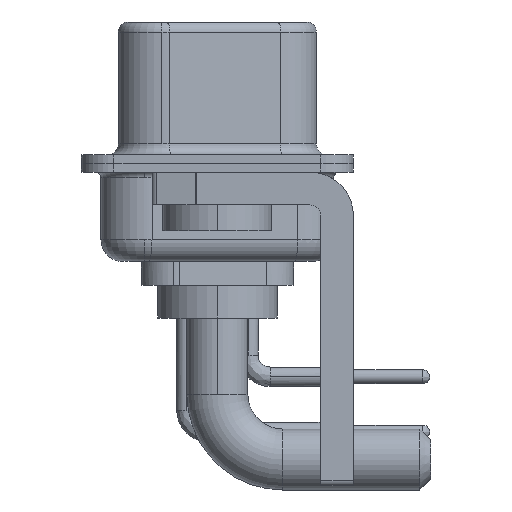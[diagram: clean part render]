
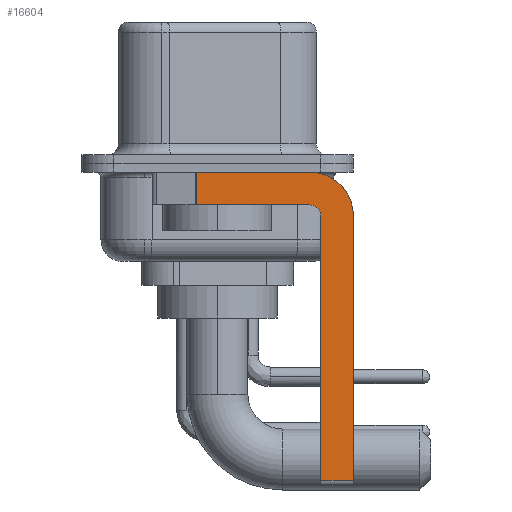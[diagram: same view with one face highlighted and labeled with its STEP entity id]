
A CAD part, left-side view. The second image highlights one B-rep face of the part: STEP entity #16604.
In plain terms, the highlighted planar face has unit normal (-1, 0, 0).
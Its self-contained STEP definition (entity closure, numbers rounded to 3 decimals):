
#209 = LINE ( 'NONE', #8824, #12988 ) ;
#269 = CARTESIAN_POINT ( 'NONE',  ( -2.9, 3., -0.4 ) ) ;
#387 = DIRECTION ( 'NONE',  ( 0., -1., 0. ) ) ;
#455 = DIRECTION ( 'NONE',  ( -1., 0., 0. ) ) ;
#853 = VECTOR ( 'NONE', #387, 1000. ) ;
#1752 = DIRECTION ( 'NONE',  ( 1., 0., 0. ) ) ;
#2207 = DIRECTION ( 'NONE',  ( 0., 0., -1. ) ) ;
#2920 = ORIENTED_EDGE ( 'NONE', *, *, #16325, .F. ) ;
#2950 = VERTEX_POINT ( 'NONE', #22799 ) ;
#3024 = FACE_OUTER_BOUND ( 'NONE', #8838, .T. ) ;
#3035 = CARTESIAN_POINT ( 'NONE',  ( -2.9, 0.978, -0.4 ) ) ;
#3582 = VERTEX_POINT ( 'NONE', #8939 ) ;
#3857 = LINE ( 'NONE', #11533, #7801 ) ;
#3875 = LINE ( 'NONE', #12969, #11647 ) ;
#4108 = ORIENTED_EDGE ( 'NONE', *, *, #15287, .F. ) ;
#4425 = DIRECTION ( 'NONE',  ( 0., 0., 1. ) ) ;
#4840 = CARTESIAN_POINT ( 'NONE',  ( -2.9, 0.978, -1.9 ) ) ;
#4851 = AXIS2_PLACEMENT_3D ( 'NONE', #7416, #1752, #12620 ) ;
#5458 = EDGE_CURVE ( 'NONE', #9371, #8896, #209, .T. ) ;
#5978 = VERTEX_POINT ( 'NONE', #4840 ) ;
#6232 = ORIENTED_EDGE ( 'NONE', *, *, #9484, .T. ) ;
#6347 = ORIENTED_EDGE ( 'NONE', *, *, #21691, .F. ) ;
#6427 = CARTESIAN_POINT ( 'NONE',  ( -2.9, -4.75, -14.8 ) ) ;
#6877 = LINE ( 'NONE', #15976, #7478 ) ;
#7175 = DIRECTION ( 'NONE',  ( 0., 0., 1. ) ) ;
#7180 = DIRECTION ( 'NONE',  ( 0., 1., 0. ) ) ;
#7416 = CARTESIAN_POINT ( 'NONE',  ( -2.9, -4.25, -2.4 ) ) ;
#7478 = VECTOR ( 'NONE', #14556, 1000. ) ;
#7801 = VECTOR ( 'NONE', #2207, 1000. ) ;
#8552 = ORIENTED_EDGE ( 'NONE', *, *, #16240, .F. ) ;
#8640 = VECTOR ( 'NONE', #4425, 1000. ) ;
#8824 = CARTESIAN_POINT ( 'NONE',  ( -2.9, -6.25, -2.4 ) ) ;
#8838 = EDGE_LOOP ( 'NONE', ( #4108, #6232, #8552, #6347, #14166, #11772, #13101, #2920 ) ) ;
#8896 = VERTEX_POINT ( 'NONE', #14082 ) ;
#8939 = CARTESIAN_POINT ( 'NONE',  ( -2.9, -4.75, -14.55 ) ) ;
#9371 = VERTEX_POINT ( 'NONE', #10715 ) ;
#9484 = EDGE_CURVE ( 'NONE', #19626, #5978, #3857, .T. ) ;
#10115 = DIRECTION ( 'NONE',  ( 0., 0., -1. ) ) ;
#10374 = EDGE_CURVE ( 'NONE', #3582, #8896, #6877, .T. ) ;
#10464 = CARTESIAN_POINT ( 'NONE',  ( -2.9, -4.25, -0.4 ) ) ;
#10715 = CARTESIAN_POINT ( 'NONE',  ( -2.9, -6.25, -2.4 ) ) ;
#11074 = DIRECTION ( 'NONE',  ( 0., 0., -1. ) ) ;
#11278 = CIRCLE ( 'NONE', #4851, 2. ) ;
#11533 = CARTESIAN_POINT ( 'NONE',  ( -2.9, 0.978, -1.9 ) ) ;
#11647 = VECTOR ( 'NONE', #7180, 1000. ) ;
#11659 = AXIS2_PLACEMENT_3D ( 'NONE', #23030, #22797, #10115 ) ;
#11772 = ORIENTED_EDGE ( 'NONE', *, *, #10374, .T. ) ;
#11863 = EDGE_CURVE ( 'NONE', #3582, #2950, #20643, .T. ) ;
#12176 = CIRCLE ( 'NONE', #15942, 0.5 ) ;
#12620 = DIRECTION ( 'NONE',  ( 0., 0., -1. ) ) ;
#12969 = CARTESIAN_POINT ( 'NONE',  ( -2.9, -4.25, -1.9 ) ) ;
#12988 = VECTOR ( 'NONE', #11074, 1000. ) ;
#13101 = ORIENTED_EDGE ( 'NONE', *, *, #5458, .F. ) ;
#14082 = CARTESIAN_POINT ( 'NONE',  ( -2.9, -6.25, -14.55 ) ) ;
#14166 = ORIENTED_EDGE ( 'NONE', *, *, #11863, .F. ) ;
#14512 = CARTESIAN_POINT ( 'NONE',  ( -2.9, -4.25, -2.4 ) ) ;
#14556 = DIRECTION ( 'NONE',  ( 0., -1., 0. ) ) ;
#15287 = EDGE_CURVE ( 'NONE', #19626, #16646, #16437, .T. ) ;
#15942 = AXIS2_PLACEMENT_3D ( 'NONE', #14512, #455, #7175 ) ;
#15976 = CARTESIAN_POINT ( 'NONE',  ( -2.9, -4.25, -14.55 ) ) ;
#16240 = EDGE_CURVE ( 'NONE', #18672, #5978, #3875, .T. ) ;
#16325 = EDGE_CURVE ( 'NONE', #16646, #9371, #11278, .T. ) ;
#16437 = LINE ( 'NONE', #269, #853 ) ;
#16604 = ADVANCED_FACE ( 'NONE', ( #3024 ), #21022, .F. ) ;
#16646 = VERTEX_POINT ( 'NONE', #10464 ) ;
#18672 = VERTEX_POINT ( 'NONE', #22177 ) ;
#19626 = VERTEX_POINT ( 'NONE', #3035 ) ;
#20643 = LINE ( 'NONE', #6427, #8640 ) ;
#21022 = PLANE ( 'NONE',  #11659 ) ;
#21691 = EDGE_CURVE ( 'NONE', #2950, #18672, #12176, .T. ) ;
#22177 = CARTESIAN_POINT ( 'NONE',  ( -2.9, -4.25, -1.9 ) ) ;
#22797 = DIRECTION ( 'NONE',  ( 1., 0., 0. ) ) ;
#22799 = CARTESIAN_POINT ( 'NONE',  ( -2.9, -4.75, -2.4 ) ) ;
#23030 = CARTESIAN_POINT ( 'NONE',  ( -2.9, -4.25, -2.4 ) ) ;
